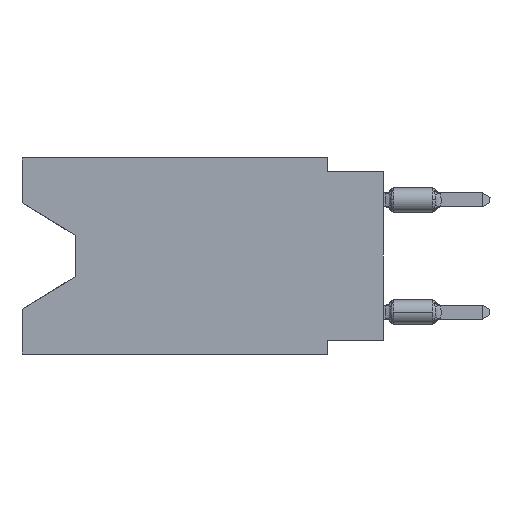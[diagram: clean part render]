
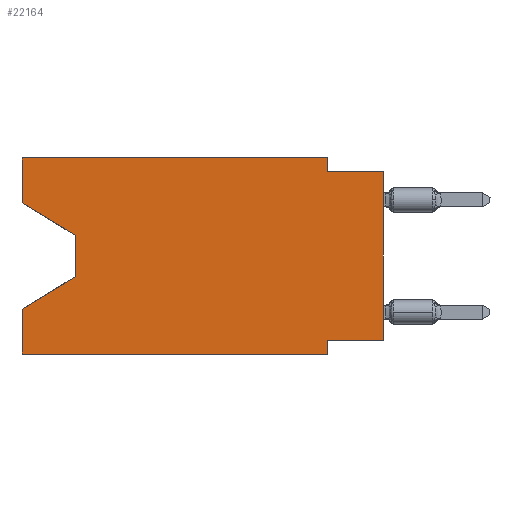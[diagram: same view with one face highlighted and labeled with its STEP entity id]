
A CAD part, left-side view. The second image highlights one B-rep face of the part: STEP entity #22164.
In plain terms, the highlighted planar face has unit normal (-1, 0, 0).
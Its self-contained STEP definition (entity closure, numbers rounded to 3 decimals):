
#17 = LINE ( 'NONE', #45380, #38077 ) ;
#124 = CARTESIAN_POINT ( 'NONE',  ( 0., 2.54, 0. ) ) ;
#561 = VECTOR ( 'NONE', #49170, 1000. ) ;
#1165 = LINE ( 'NONE', #55673, #28558 ) ;
#1824 = DIRECTION ( 'NONE',  ( 0., 0., 1. ) ) ;
#5075 = CARTESIAN_POINT ( 'NONE',  ( 0., 16.383, 0. ) ) ;
#6134 = LINE ( 'NONE', #40726, #55344 ) ;
#7775 = VERTEX_POINT ( 'NONE', #47970 ) ;
#10757 = CARTESIAN_POINT ( 'NONE',  ( 0., 16.383, -2.038 ) ) ;
#11081 = DIRECTION ( 'NONE',  ( 0., -0.855, -0.519 ) ) ;
#12944 = EDGE_CURVE ( 'NONE', #27041, #17736, #29568, .T. ) ;
#13185 = CARTESIAN_POINT ( 'NONE',  ( 0., 0., -8.255 ) ) ;
#14233 = ORIENTED_EDGE ( 'NONE', *, *, #45882, .T. ) ;
#14751 = VECTOR ( 'NONE', #30499, 1000. ) ;
#15170 = ORIENTED_EDGE ( 'NONE', *, *, #44887, .F. ) ;
#15274 = VECTOR ( 'NONE', #57354, 1000. ) ;
#15428 = VECTOR ( 'NONE', #11081, 1000. ) ;
#16715 = CARTESIAN_POINT ( 'NONE',  ( 0., 16.383, -8.89 ) ) ;
#16859 = LINE ( 'NONE', #62578, #15274 ) ;
#17223 = ORIENTED_EDGE ( 'NONE', *, *, #36226, .T. ) ;
#17736 = VERTEX_POINT ( 'NONE', #34444 ) ;
#18023 = DIRECTION ( 'NONE',  ( 0., 0., -1. ) ) ;
#21519 = CARTESIAN_POINT ( 'NONE',  ( 0., 16.383, -8.89 ) ) ;
#21604 = EDGE_CURVE ( 'NONE', #54706, #35481, #6134, .T. ) ;
#21769 = CARTESIAN_POINT ( 'NONE',  ( 0., 16.383, 0. ) ) ;
#22119 = ORIENTED_EDGE ( 'NONE', *, *, #32358, .F. ) ;
#22164 = ADVANCED_FACE ( 'NONE', ( #49782 ), #53711, .F. ) ;
#22611 = CARTESIAN_POINT ( 'NONE',  ( 0., 0., 0. ) ) ;
#24326 = DIRECTION ( 'NONE',  ( 0., 0., -1. ) ) ;
#24473 = ORIENTED_EDGE ( 'NONE', *, *, #46283, .T. ) ;
#26075 = ORIENTED_EDGE ( 'NONE', *, *, #37333, .T. ) ;
#27041 = VERTEX_POINT ( 'NONE', #21769 ) ;
#27993 = VERTEX_POINT ( 'NONE', #33322 ) ;
#28335 = EDGE_CURVE ( 'NONE', #27993, #33222, #16859, .T. ) ;
#28558 = VECTOR ( 'NONE', #1824, 1000. ) ;
#28678 = CARTESIAN_POINT ( 'NONE',  ( 0., 2.54, -8.255 ) ) ;
#29568 = LINE ( 'NONE', #38431, #561 ) ;
#29742 = DIRECTION ( 'NONE',  ( 0., 0., -1. ) ) ;
#30499 = DIRECTION ( 'NONE',  ( 0., 0., 1. ) ) ;
#30590 = DIRECTION ( 'NONE',  ( 0., 0.855, -0.519 ) ) ;
#31133 = EDGE_CURVE ( 'NONE', #34967, #35481, #56286, .T. ) ;
#32358 = EDGE_CURVE ( 'NONE', #39588, #27041, #1165, .T. ) ;
#33222 = VERTEX_POINT ( 'NONE', #45422 ) ;
#33322 = CARTESIAN_POINT ( 'NONE',  ( 0., 2.54, -0.635 ) ) ;
#34012 = EDGE_CURVE ( 'NONE', #34589, #59886, #17, .T. ) ;
#34444 = CARTESIAN_POINT ( 'NONE',  ( 0., 2.54, 0. ) ) ;
#34447 = DIRECTION ( 'NONE',  ( 1., 0., 0. ) ) ;
#34589 = VERTEX_POINT ( 'NONE', #13185 ) ;
#34967 = VERTEX_POINT ( 'NONE', #16715 ) ;
#35481 = VERTEX_POINT ( 'NONE', #47967 ) ;
#35844 = ORIENTED_EDGE ( 'NONE', *, *, #12944, .F. ) ;
#35895 = LINE ( 'NONE', #10757, #15428 ) ;
#36213 = VECTOR ( 'NONE', #61366, 1000. ) ;
#36226 = EDGE_CURVE ( 'NONE', #34967, #44186, #51219, .T. ) ;
#37333 = EDGE_CURVE ( 'NONE', #39588, #7775, #35895, .T. ) ;
#38077 = VECTOR ( 'NONE', #49953, 1000. ) ;
#38431 = CARTESIAN_POINT ( 'NONE',  ( 0., 16.383, 0. ) ) ;
#39562 = CARTESIAN_POINT ( 'NONE',  ( 0., 13.97, -3.505 ) ) ;
#39588 = VERTEX_POINT ( 'NONE', #40594 ) ;
#40594 = CARTESIAN_POINT ( 'NONE',  ( 0., 16.383, -2.038 ) ) ;
#40726 = CARTESIAN_POINT ( 'NONE',  ( 0., 13.97, -5.385 ) ) ;
#42831 = LINE ( 'NONE', #62758, #47877 ) ;
#43887 = LINE ( 'NONE', #124, #64406 ) ;
#44186 = VERTEX_POINT ( 'NONE', #44602 ) ;
#44452 = LINE ( 'NONE', #39562, #63229 ) ;
#44602 = CARTESIAN_POINT ( 'NONE',  ( 0., 2.54, -8.89 ) ) ;
#44887 = EDGE_CURVE ( 'NONE', #59886, #44186, #42831, .T. ) ;
#45380 = CARTESIAN_POINT ( 'NONE',  ( 0., 0., -8.255 ) ) ;
#45422 = CARTESIAN_POINT ( 'NONE',  ( 0., 0., -0.635 ) ) ;
#45882 = EDGE_CURVE ( 'NONE', #34589, #33222, #46452, .T. ) ;
#46283 = EDGE_CURVE ( 'NONE', #7775, #54706, #44452, .T. ) ;
#46452 = LINE ( 'NONE', #22611, #50633 ) ;
#47570 = ORIENTED_EDGE ( 'NONE', *, *, #34012, .F. ) ;
#47877 = VECTOR ( 'NONE', #18023, 1000. ) ;
#47967 = CARTESIAN_POINT ( 'NONE',  ( 0., 16.383, -6.852 ) ) ;
#47970 = CARTESIAN_POINT ( 'NONE',  ( 0., 13.97, -3.505 ) ) ;
#49170 = DIRECTION ( 'NONE',  ( 0., -1., 0. ) ) ;
#49581 = ORIENTED_EDGE ( 'NONE', *, *, #61938, .F. ) ;
#49782 = FACE_OUTER_BOUND ( 'NONE', #50993, .T. ) ;
#49953 = DIRECTION ( 'NONE',  ( 0., 1., 0. ) ) ;
#50633 = VECTOR ( 'NONE', #51347, 1000. ) ;
#50993 = EDGE_LOOP ( 'NONE', ( #26075, #24473, #55355, #60691, #17223, #15170, #47570, #14233, #55448, #49581, #35844, #22119 ) ) ;
#51219 = LINE ( 'NONE', #21519, #36213 ) ;
#51347 = DIRECTION ( 'NONE',  ( 0., 0., 1. ) ) ;
#53711 = PLANE ( 'NONE',  #57556 ) ;
#54706 = VERTEX_POINT ( 'NONE', #63420 ) ;
#55344 = VECTOR ( 'NONE', #30590, 1000. ) ;
#55355 = ORIENTED_EDGE ( 'NONE', *, *, #21604, .T. ) ;
#55448 = ORIENTED_EDGE ( 'NONE', *, *, #28335, .F. ) ;
#55673 = CARTESIAN_POINT ( 'NONE',  ( 0., 16.383, 0. ) ) ;
#56286 = LINE ( 'NONE', #60558, #14751 ) ;
#57354 = DIRECTION ( 'NONE',  ( 0., -1., 0. ) ) ;
#57556 = AXIS2_PLACEMENT_3D ( 'NONE', #5075, #34447, #24326 ) ;
#59886 = VERTEX_POINT ( 'NONE', #28678 ) ;
#60558 = CARTESIAN_POINT ( 'NONE',  ( 0., 16.383, 0. ) ) ;
#60691 = ORIENTED_EDGE ( 'NONE', *, *, #31133, .F. ) ;
#61366 = DIRECTION ( 'NONE',  ( 0., -1., 0. ) ) ;
#61938 = EDGE_CURVE ( 'NONE', #17736, #27993, #43887, .T. ) ;
#62578 = CARTESIAN_POINT ( 'NONE',  ( 0., 0., -0.635 ) ) ;
#62758 = CARTESIAN_POINT ( 'NONE',  ( 0., 2.54, -8.89 ) ) ;
#63229 = VECTOR ( 'NONE', #29742, 1000. ) ;
#63420 = CARTESIAN_POINT ( 'NONE',  ( 0., 13.97, -5.385 ) ) ;
#63819 = DIRECTION ( 'NONE',  ( 0., 0., -1. ) ) ;
#64406 = VECTOR ( 'NONE', #63819, 1000. ) ;
